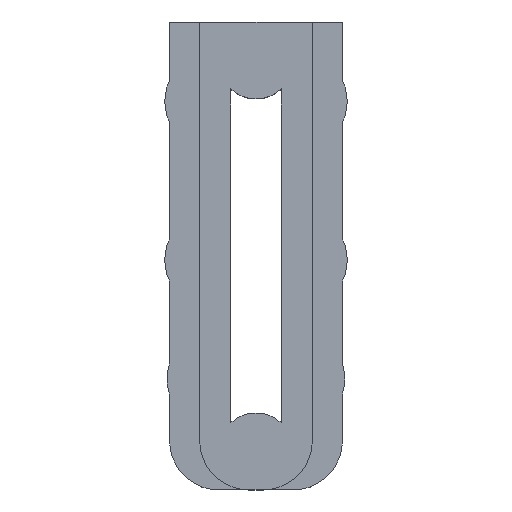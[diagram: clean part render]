
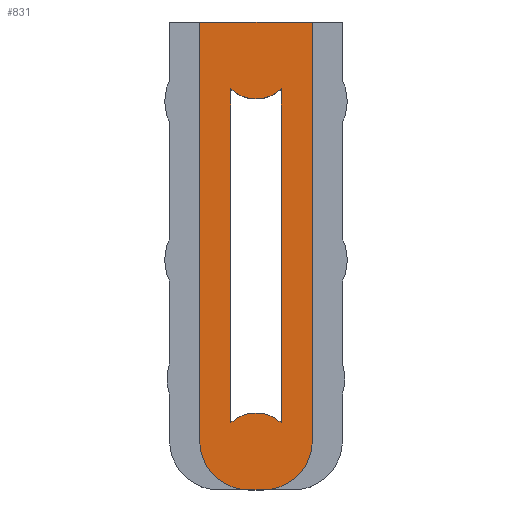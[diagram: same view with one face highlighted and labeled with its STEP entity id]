
A CAD part, top view. The second image highlights one B-rep face of the part: STEP entity #831.
In plain terms, the highlighted planar face has unit normal (0, 0, 1).
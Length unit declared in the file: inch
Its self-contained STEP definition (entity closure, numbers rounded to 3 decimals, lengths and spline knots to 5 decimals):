
#5 = VECTOR ( 'NONE', #101, 39.37008 ) ;
#10 = VERTEX_POINT ( 'NONE', #806 ) ;
#36 = PLANE ( 'NONE',  #1330 ) ;
#66 = CIRCLE ( 'NONE', #825, 0.031 ) ;
#78 = EDGE_LOOP ( 'NONE', ( #120, #1320, #421, #167 ) ) ;
#93 = CARTESIAN_POINT ( 'NONE',  ( 0.0045, -0.1165, 0.0175 ) ) ;
#101 = DIRECTION ( 'NONE',  ( 0., -1., 0. ) ) ;
#115 = LINE ( 'NONE', #300, #583 ) ;
#120 = ORIENTED_EDGE ( 'NONE', *, *, #134, .F. ) ;
#134 = EDGE_CURVE ( 'NONE', #10, #194, #645, .T. ) ;
#137 = CIRCLE ( 'NONE', #1061, 0.0235 ) ;
#160 = EDGE_CURVE ( 'NONE', #936, #693, #972, .T. ) ;
#167 = ORIENTED_EDGE ( 'NONE', *, *, #1230, .F. ) ;
#179 = VECTOR ( 'NONE', #381, 39.37008 ) ;
#194 = VERTEX_POINT ( 'NONE', #332 ) ;
#204 = CIRCLE ( 'NONE', #849, 0.0235 ) ;
#207 = ORIENTED_EDGE ( 'NONE', *, *, #160, .F. ) ;
#225 = VECTOR ( 'NONE', #1169, 39.37008 ) ;
#271 = CARTESIAN_POINT ( 'NONE',  ( -0.016, -0.10529, 0.0175 ) ) ;
#278 = DIRECTION ( 'NONE',  ( 0., 0., -1. ) ) ;
#283 = EDGE_CURVE ( 'NONE', #1229, #936, #66, .T. ) ;
#293 = VECTOR ( 'NONE', #682, 39.37008 ) ;
#295 = DIRECTION ( 'NONE',  ( 0., 0., -1. ) ) ;
#300 = CARTESIAN_POINT ( 'NONE',  ( -0.0545, 0.1475, 0.0175 ) ) ;
#310 = CIRCLE ( 'NONE', #674, 0.031 ) ;
#313 = VERTEX_POINT ( 'NONE', #271 ) ;
#332 = CARTESIAN_POINT ( 'NONE',  ( 0.016, 0.10529, 0.0175 ) ) ;
#361 = VERTEX_POINT ( 'NONE', #1296 ) ;
#368 = ORIENTED_EDGE ( 'NONE', *, *, #380, .T. ) ;
#380 = EDGE_CURVE ( 'NONE', #813, #361, #395, .T. ) ;
#381 = DIRECTION ( 'NONE',  ( 0., 1., 0. ) ) ;
#395 = LINE ( 'NONE', #900, #179 ) ;
#421 = ORIENTED_EDGE ( 'NONE', *, *, #1197, .F. ) ;
#432 = EDGE_CURVE ( 'NONE', #813, #1141, #310, .T. ) ;
#436 = CARTESIAN_POINT ( 'NONE',  ( 0.016, -0.10529, 0.0175 ) ) ;
#477 = ORIENTED_EDGE ( 'NONE', *, *, #432, .F. ) ;
#479 = EDGE_CURVE ( 'NONE', #313, #10, #204, .T. ) ;
#485 = VERTEX_POINT ( 'NONE', #817 ) ;
#506 = DIRECTION ( 'NONE',  ( 0., 0., -1. ) ) ;
#509 = DIRECTION ( 'NONE',  ( 0., 0., -1. ) ) ;
#522 = CARTESIAN_POINT ( 'NONE',  ( -0.016, 0.10529, 0.0175 ) ) ;
#553 = FACE_BOUND ( 'NONE', #78, .T. ) ;
#581 = CARTESIAN_POINT ( 'NONE',  ( -0.0235, -0.1475, 0.0175 ) ) ;
#583 = VECTOR ( 'NONE', #799, 39.37008 ) ;
#609 = DIRECTION ( 'NONE',  ( -1., 0., 0. ) ) ;
#610 = EDGE_CURVE ( 'NONE', #1229, #1141, #1201, .T. ) ;
#643 = CARTESIAN_POINT ( 'NONE',  ( -0.0355, -0.1165, 0.0175 ) ) ;
#645 = LINE ( 'NONE', #436, #1133 ) ;
#656 = DIRECTION ( 'NONE',  ( 0., 1., 0. ) ) ;
#674 = AXIS2_PLACEMENT_3D ( 'NONE', #93, #509, #1321 ) ;
#682 = DIRECTION ( 'NONE',  ( 1., 0., 0. ) ) ;
#693 = VERTEX_POINT ( 'NONE', #1045 ) ;
#730 = DIRECTION ( 'NONE',  ( 1., 0., 0. ) ) ;
#762 = DIRECTION ( 'NONE',  ( 0., 0., 1. ) ) ;
#767 = CARTESIAN_POINT ( 'NONE',  ( 0.0355, -0.1165, 0.0175 ) ) ;
#779 = DIRECTION ( 'NONE',  ( 1., 0., 0. ) ) ;
#799 = DIRECTION ( 'NONE',  ( -1., 0., 0. ) ) ;
#806 = CARTESIAN_POINT ( 'NONE',  ( 0.016, -0.10529, 0.0175 ) ) ;
#813 = VERTEX_POINT ( 'NONE', #767 ) ;
#817 = CARTESIAN_POINT ( 'NONE',  ( -0.016, 0.10529, 0.0175 ) ) ;
#825 = AXIS2_PLACEMENT_3D ( 'NONE', #1272, #278, #779 ) ;
#831 = ADVANCED_FACE ( 'NONE', ( #1062, #553 ), #36, .T. ) ;
#849 = AXIS2_PLACEMENT_3D ( 'NONE', #908, #295, #609 ) ;
#853 = EDGE_LOOP ( 'NONE', ( #1024, #1003, #477, #368, #1281, #207 ) ) ;
#859 = CARTESIAN_POINT ( 'NONE',  ( -0.0355, -0.1475, 0.0175 ) ) ;
#860 = CARTESIAN_POINT ( 'NONE',  ( -0.0265, 0.0975, 0.0175 ) ) ;
#900 = CARTESIAN_POINT ( 'NONE',  ( 0.0355, -0.1475, 0.0175 ) ) ;
#908 = CARTESIAN_POINT ( 'NONE',  ( 0., -0.1225, 0.0175 ) ) ;
#936 = VERTEX_POINT ( 'NONE', #643 ) ;
#972 = LINE ( 'NONE', #859, #225 ) ;
#1003 = ORIENTED_EDGE ( 'NONE', *, *, #610, .T. ) ;
#1007 = CARTESIAN_POINT ( 'NONE',  ( 0.0045, -0.1475, 0.0175 ) ) ;
#1023 = LINE ( 'NONE', #522, #5 ) ;
#1024 = ORIENTED_EDGE ( 'NONE', *, *, #283, .F. ) ;
#1033 = CARTESIAN_POINT ( 'NONE',  ( -0.0045, -0.1475, 0.0175 ) ) ;
#1045 = CARTESIAN_POINT ( 'NONE',  ( -0.0355, 0.1475, 0.0175 ) ) ;
#1061 = AXIS2_PLACEMENT_3D ( 'NONE', #1336, #506, #730 ) ;
#1062 = FACE_OUTER_BOUND ( 'NONE', #853, .T. ) ;
#1133 = VECTOR ( 'NONE', #656, 39.37008 ) ;
#1141 = VERTEX_POINT ( 'NONE', #1007 ) ;
#1169 = DIRECTION ( 'NONE',  ( 0., 1., 0. ) ) ;
#1171 = DIRECTION ( 'NONE',  ( 1., 0., 0. ) ) ;
#1197 = EDGE_CURVE ( 'NONE', #485, #313, #1023, .T. ) ;
#1201 = LINE ( 'NONE', #581, #293 ) ;
#1229 = VERTEX_POINT ( 'NONE', #1033 ) ;
#1230 = EDGE_CURVE ( 'NONE', #194, #485, #137, .T. ) ;
#1238 = EDGE_CURVE ( 'NONE', #361, #693, #115, .T. ) ;
#1272 = CARTESIAN_POINT ( 'NONE',  ( -0.0045, -0.1165, 0.0175 ) ) ;
#1281 = ORIENTED_EDGE ( 'NONE', *, *, #1238, .T. ) ;
#1296 = CARTESIAN_POINT ( 'NONE',  ( 0.0355, 0.1475, 0.0175 ) ) ;
#1320 = ORIENTED_EDGE ( 'NONE', *, *, #479, .F. ) ;
#1321 = DIRECTION ( 'NONE',  ( -1., 0., 0. ) ) ;
#1330 = AXIS2_PLACEMENT_3D ( 'NONE', #860, #762, #1171 ) ;
#1336 = CARTESIAN_POINT ( 'NONE',  ( 0., 0.1225, 0.0175 ) ) ;
